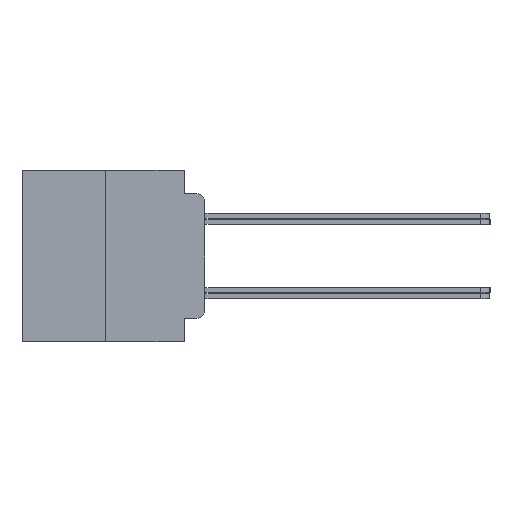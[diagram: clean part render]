
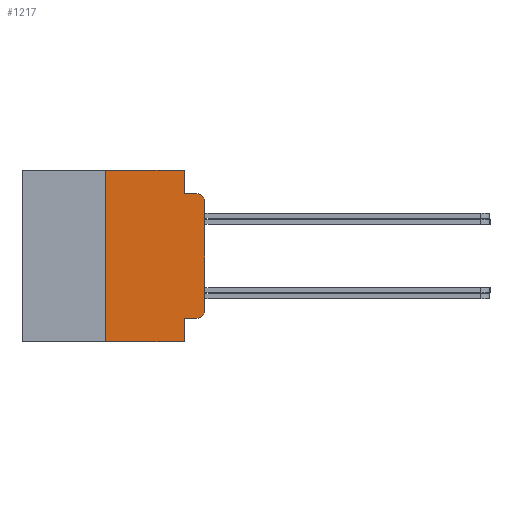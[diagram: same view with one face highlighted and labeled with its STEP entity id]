
A CAD part, left-side view. The second image highlights one B-rep face of the part: STEP entity #1217.
In plain terms, the highlighted planar face has unit normal (-1, 0, 0).
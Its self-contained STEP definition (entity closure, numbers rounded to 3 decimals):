
#37 = LINE ( 'NONE', #22099, #1084 ) ;
#501 = ORIENTED_EDGE ( 'NONE', *, *, #10188, .T. ) ;
#936 = CARTESIAN_POINT ( 'NONE',  ( -75.603, 1.295, 5.486 ) ) ;
#1084 = VECTOR ( 'NONE', #24284, 1000. ) ;
#1096 = ORIENTED_EDGE ( 'NONE', *, *, #16506, .F. ) ;
#1217 = ADVANCED_FACE ( 'NONE', ( #26942 ), #12998, .F. ) ;
#1580 = ORIENTED_EDGE ( 'NONE', *, *, #21860, .T. ) ;
#1838 = DIRECTION ( 'NONE',  ( 0., -1., 0. ) ) ;
#2126 = VECTOR ( 'NONE', #1838, 1000. ) ;
#2975 = CARTESIAN_POINT ( 'NONE',  ( -75.603, 0.508, -3.975 ) ) ;
#3009 = LINE ( 'NONE', #13217, #23348 ) ;
#3736 = ORIENTED_EDGE ( 'NONE', *, *, #12303, .F. ) ;
#4040 = CARTESIAN_POINT ( 'NONE',  ( -75.603, 6.35, -5.486 ) ) ;
#4196 = LINE ( 'NONE', #12856, #2126 ) ;
#4206 = DIRECTION ( 'NONE',  ( 0., 0., -1. ) ) ;
#4378 = VECTOR ( 'NONE', #26392, 1000. ) ;
#4614 = ORIENTED_EDGE ( 'NONE', *, *, #22035, .F. ) ;
#4713 = DIRECTION ( 'NONE',  ( 0., -1., 0. ) ) ;
#5086 = EDGE_CURVE ( 'NONE', #5783, #5306, #10258, .T. ) ;
#5306 = VERTEX_POINT ( 'NONE', #20645 ) ;
#5783 = VERTEX_POINT ( 'NONE', #7013 ) ;
#6335 = DIRECTION ( 'NONE',  ( 1., 0., 0. ) ) ;
#6758 = LINE ( 'NONE', #26856, #8146 ) ;
#6822 = ORIENTED_EDGE ( 'NONE', *, *, #26743, .T. ) ;
#7013 = CARTESIAN_POINT ( 'NONE',  ( -75.603, 1.295, -3.975 ) ) ;
#7328 = ORIENTED_EDGE ( 'NONE', *, *, #24906, .F. ) ;
#7957 = CARTESIAN_POINT ( 'NONE',  ( -75.603, 6.35, 5.486 ) ) ;
#8082 = CARTESIAN_POINT ( 'NONE',  ( -75.603, 1.295, 3.975 ) ) ;
#8146 = VECTOR ( 'NONE', #18223, 1000. ) ;
#8905 = ORIENTED_EDGE ( 'NONE', *, *, #19605, .T. ) ;
#9200 = VERTEX_POINT ( 'NONE', #21459 ) ;
#10072 = CARTESIAN_POINT ( 'NONE',  ( -75.603, 6.35, -5.486 ) ) ;
#10188 = EDGE_CURVE ( 'NONE', #25193, #16894, #22514, .T. ) ;
#10258 = LINE ( 'NONE', #17565, #4378 ) ;
#10656 = VERTEX_POINT ( 'NONE', #23512 ) ;
#11874 = DIRECTION ( 'NONE',  ( 0., 0., -1. ) ) ;
#12303 = EDGE_CURVE ( 'NONE', #28511, #15435, #37, .T. ) ;
#12380 = DIRECTION ( 'NONE',  ( 0., 0., -1. ) ) ;
#12472 = DIRECTION ( 'NONE',  ( -1., 0., 0. ) ) ;
#12569 = CARTESIAN_POINT ( 'NONE',  ( -75.603, 0.508, 3.467 ) ) ;
#12734 = EDGE_CURVE ( 'NONE', #23861, #5306, #3009, .T. ) ;
#12856 = CARTESIAN_POINT ( 'NONE',  ( -75.603, 11.684, 5.486 ) ) ;
#12998 = PLANE ( 'NONE',  #21403 ) ;
#13048 = DIRECTION ( 'NONE',  ( 0., -1., 0. ) ) ;
#13217 = CARTESIAN_POINT ( 'NONE',  ( -75.603, 11.684, -5.486 ) ) ;
#15167 = CARTESIAN_POINT ( 'NONE',  ( -75.603, 1.295, 3.975 ) ) ;
#15435 = VERTEX_POINT ( 'NONE', #8082 ) ;
#15668 = ORIENTED_EDGE ( 'NONE', *, *, #12734, .T. ) ;
#15820 = VECTOR ( 'NONE', #20292, 1000. ) ;
#16039 = VERTEX_POINT ( 'NONE', #7957 ) ;
#16506 = EDGE_CURVE ( 'NONE', #16039, #28511, #4196, .T. ) ;
#16894 = VERTEX_POINT ( 'NONE', #16895 ) ;
#16895 = CARTESIAN_POINT ( 'NONE',  ( -75.603, 0., -3.467 ) ) ;
#17334 = CARTESIAN_POINT ( 'NONE',  ( -75.603, 11.684, 5.486 ) ) ;
#17565 = CARTESIAN_POINT ( 'NONE',  ( -75.603, 1.295, 0. ) ) ;
#18223 = DIRECTION ( 'NONE',  ( 0., -1., 0. ) ) ;
#19605 = EDGE_CURVE ( 'NONE', #16894, #9200, #27863, .T. ) ;
#19637 = AXIS2_PLACEMENT_3D ( 'NONE', #25041, #27362, #11874 ) ;
#20292 = DIRECTION ( 'NONE',  ( 0., 0., 1. ) ) ;
#20342 = LINE ( 'NONE', #10072, #27557 ) ;
#20645 = CARTESIAN_POINT ( 'NONE',  ( -75.603, 1.295, -5.486 ) ) ;
#20859 = VECTOR ( 'NONE', #13048, 1000. ) ;
#20883 = CIRCLE ( 'NONE', #26101, 0.508 ) ;
#21403 = AXIS2_PLACEMENT_3D ( 'NONE', #17334, #6335, #4206 ) ;
#21459 = CARTESIAN_POINT ( 'NONE',  ( -75.603, 0., 3.467 ) ) ;
#21860 = EDGE_CURVE ( 'NONE', #9200, #10656, #20883, .T. ) ;
#22035 = EDGE_CURVE ( 'NONE', #15435, #10656, #26685, .T. ) ;
#22099 = CARTESIAN_POINT ( 'NONE',  ( -75.603, 1.295, 0. ) ) ;
#22115 = CARTESIAN_POINT ( 'NONE',  ( -75.603, 0., 5.486 ) ) ;
#22514 = CIRCLE ( 'NONE', #19637, 0.508 ) ;
#23348 = VECTOR ( 'NONE', #4713, 1000. ) ;
#23512 = CARTESIAN_POINT ( 'NONE',  ( -75.603, 0.508, 3.975 ) ) ;
#23861 = VERTEX_POINT ( 'NONE', #4040 ) ;
#24284 = DIRECTION ( 'NONE',  ( 0., 0., -1. ) ) ;
#24906 = EDGE_CURVE ( 'NONE', #23861, #16039, #20342, .T. ) ;
#25041 = CARTESIAN_POINT ( 'NONE',  ( -75.603, 0.508, -3.467 ) ) ;
#25193 = VERTEX_POINT ( 'NONE', #2975 ) ;
#25470 = DIRECTION ( 'NONE',  ( 0., 0., 1. ) ) ;
#26101 = AXIS2_PLACEMENT_3D ( 'NONE', #12569, #12472, #12380 ) ;
#26208 = EDGE_LOOP ( 'NONE', ( #6822, #501, #8905, #1580, #4614, #3736, #1096, #7328, #15668, #26756 ) ) ;
#26392 = DIRECTION ( 'NONE',  ( 0., 0., -1. ) ) ;
#26685 = LINE ( 'NONE', #15167, #20859 ) ;
#26743 = EDGE_CURVE ( 'NONE', #5783, #25193, #6758, .T. ) ;
#26756 = ORIENTED_EDGE ( 'NONE', *, *, #5086, .F. ) ;
#26856 = CARTESIAN_POINT ( 'NONE',  ( -75.603, 1.295, -3.975 ) ) ;
#26942 = FACE_OUTER_BOUND ( 'NONE', #26208, .T. ) ;
#27362 = DIRECTION ( 'NONE',  ( -1., 0., 0. ) ) ;
#27557 = VECTOR ( 'NONE', #25470, 1000. ) ;
#27863 = LINE ( 'NONE', #22115, #15820 ) ;
#28511 = VERTEX_POINT ( 'NONE', #936 ) ;
